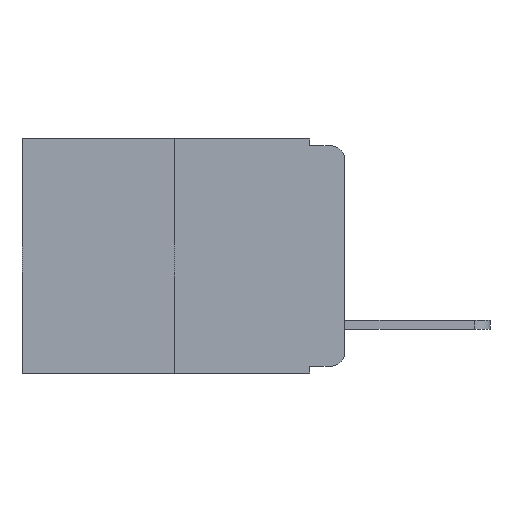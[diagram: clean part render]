
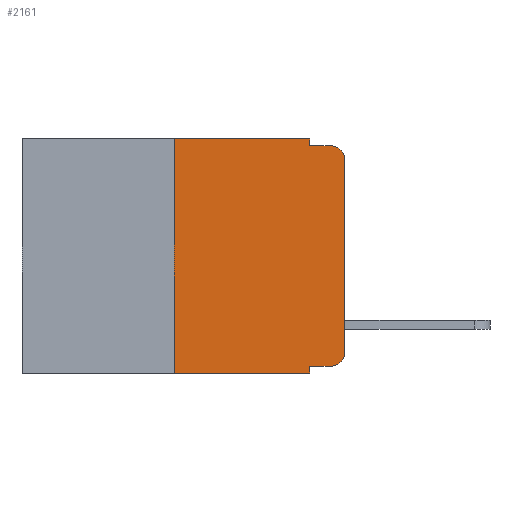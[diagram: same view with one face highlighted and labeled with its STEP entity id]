
A CAD part, left-side view. The second image highlights one B-rep face of the part: STEP entity #2161.
In plain terms, the highlighted planar face has unit normal (-1, 0, 0).
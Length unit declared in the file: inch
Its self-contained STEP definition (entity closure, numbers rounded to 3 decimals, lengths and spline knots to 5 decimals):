
#366 = VERTEX_POINT ( 'NONE', #12138 ) ;
#559 = DIRECTION ( 'NONE',  ( 0., -1., 0. ) ) ;
#1213 = VECTOR ( 'NONE', #559, 39.37008 ) ;
#1347 = CARTESIAN_POINT ( 'NONE',  ( 0., 0.051, -0.01 ) ) ;
#1395 = CARTESIAN_POINT ( 'NONE',  ( 0., 0.02, -0.03 ) ) ;
#1619 = CARTESIAN_POINT ( 'NONE',  ( 0., 0.25, 0. ) ) ;
#1720 = LINE ( 'NONE', #11743, #8694 ) ;
#1754 = DIRECTION ( 'NONE',  ( 1., 0., 0. ) ) ;
#1811 = LINE ( 'NONE', #12158, #14502 ) ;
#1887 = CARTESIAN_POINT ( 'NONE',  ( 0., 0.02, -0.01 ) ) ;
#2161 = ADVANCED_FACE ( 'NONE', ( #7133 ), #8651, .F. ) ;
#2276 = DIRECTION ( 'NONE',  ( -1., 0., 0. ) ) ;
#2451 = VECTOR ( 'NONE', #3055, 39.37008 ) ;
#2635 = DIRECTION ( 'NONE',  ( 0., 0., -1. ) ) ;
#2813 = DIRECTION ( 'NONE',  ( 0., 0., -1. ) ) ;
#2818 = VECTOR ( 'NONE', #8005, 39.37008 ) ;
#3055 = DIRECTION ( 'NONE',  ( 0., 0., -1. ) ) ;
#3097 = EDGE_CURVE ( 'NONE', #13874, #5766, #4501, .T. ) ;
#3122 = ORIENTED_EDGE ( 'NONE', *, *, #5126, .T. ) ;
#3855 = VECTOR ( 'NONE', #10540, 39.37008 ) ;
#3976 = EDGE_CURVE ( 'NONE', #11654, #7287, #7763, .T. ) ;
#4277 = VECTOR ( 'NONE', #8811, 39.37008 ) ;
#4360 = DIRECTION ( 'NONE',  ( 0., 0., 1. ) ) ;
#4501 = LINE ( 'NONE', #1347, #1213 ) ;
#4896 = VERTEX_POINT ( 'NONE', #12552 ) ;
#5019 = AXIS2_PLACEMENT_3D ( 'NONE', #7340, #1754, #2813 ) ;
#5088 = CARTESIAN_POINT ( 'NONE',  ( 0., 0.473, -0.343 ) ) ;
#5126 = EDGE_CURVE ( 'NONE', #366, #11071, #10782, .T. ) ;
#5196 = CARTESIAN_POINT ( 'NONE',  ( 0., 0.25, -0.343 ) ) ;
#5318 = EDGE_CURVE ( 'NONE', #11071, #7350, #14222, .T. ) ;
#5589 = AXIS2_PLACEMENT_3D ( 'NONE', #1395, #10014, #2635 ) ;
#5659 = ORIENTED_EDGE ( 'NONE', *, *, #10880, .F. ) ;
#5766 = VERTEX_POINT ( 'NONE', #1887 ) ;
#6203 = ORIENTED_EDGE ( 'NONE', *, *, #13486, .T. ) ;
#6761 = CARTESIAN_POINT ( 'NONE',  ( 0., 0.051, 0. ) ) ;
#7133 = FACE_OUTER_BOUND ( 'NONE', #9775, .T. ) ;
#7287 = VERTEX_POINT ( 'NONE', #13765 ) ;
#7340 = CARTESIAN_POINT ( 'NONE',  ( 0., 0.473, 0. ) ) ;
#7350 = VERTEX_POINT ( 'NONE', #8985 ) ;
#7395 = ORIENTED_EDGE ( 'NONE', *, *, #3976, .F. ) ;
#7576 = LINE ( 'NONE', #5088, #4277 ) ;
#7763 = LINE ( 'NONE', #8112, #13898 ) ;
#7936 = CIRCLE ( 'NONE', #5589, 0.02 ) ;
#8005 = DIRECTION ( 'NONE',  ( 0., 0., -1. ) ) ;
#8017 = EDGE_CURVE ( 'NONE', #366, #9516, #12270, .T. ) ;
#8112 = CARTESIAN_POINT ( 'NONE',  ( 0., 0.473, 0. ) ) ;
#8351 = ORIENTED_EDGE ( 'NONE', *, *, #12646, .T. ) ;
#8651 = PLANE ( 'NONE',  #5019 ) ;
#8694 = VECTOR ( 'NONE', #4360, 39.37008 ) ;
#8746 = AXIS2_PLACEMENT_3D ( 'NONE', #9675, #2276, #10911 ) ;
#8811 = DIRECTION ( 'NONE',  ( 0., -1., 0. ) ) ;
#8833 = ORIENTED_EDGE ( 'NONE', *, *, #8017, .F. ) ;
#8985 = CARTESIAN_POINT ( 'NONE',  ( 0., 0., -0.313 ) ) ;
#9018 = LINE ( 'NONE', #6761, #2451 ) ;
#9309 = CARTESIAN_POINT ( 'NONE',  ( 0., 0.051, -0.333 ) ) ;
#9392 = CARTESIAN_POINT ( 'NONE',  ( 0., 0.051, -0.343 ) ) ;
#9422 = EDGE_CURVE ( 'NONE', #7287, #13874, #9018, .T. ) ;
#9516 = VERTEX_POINT ( 'NONE', #9392 ) ;
#9675 = CARTESIAN_POINT ( 'NONE',  ( 0., 0.02, -0.313 ) ) ;
#9775 = EDGE_LOOP ( 'NONE', ( #6203, #12800, #14505, #10079, #7395, #5659, #8351, #8833, #3122, #11306 ) ) ;
#10014 = DIRECTION ( 'NONE',  ( -1., 0., 0. ) ) ;
#10079 = ORIENTED_EDGE ( 'NONE', *, *, #9422, .F. ) ;
#10540 = DIRECTION ( 'NONE',  ( 0., -1., 0. ) ) ;
#10782 = LINE ( 'NONE', #9309, #3855 ) ;
#10880 = EDGE_CURVE ( 'NONE', #11084, #11654, #1811, .T. ) ;
#10911 = DIRECTION ( 'NONE',  ( 0., 0., -1. ) ) ;
#11071 = VERTEX_POINT ( 'NONE', #11347 ) ;
#11084 = VERTEX_POINT ( 'NONE', #5196 ) ;
#11306 = ORIENTED_EDGE ( 'NONE', *, *, #5318, .T. ) ;
#11347 = CARTESIAN_POINT ( 'NONE',  ( 0., 0.02, -0.333 ) ) ;
#11654 = VERTEX_POINT ( 'NONE', #1619 ) ;
#11743 = CARTESIAN_POINT ( 'NONE',  ( 0., 0., 0. ) ) ;
#12138 = CARTESIAN_POINT ( 'NONE',  ( 0., 0.051, -0.333 ) ) ;
#12158 = CARTESIAN_POINT ( 'NONE',  ( 0., 0.25, 0. ) ) ;
#12270 = LINE ( 'NONE', #15317, #2818 ) ;
#12552 = CARTESIAN_POINT ( 'NONE',  ( 0., 0., -0.03 ) ) ;
#12593 = CARTESIAN_POINT ( 'NONE',  ( 0., 0.051, -0.01 ) ) ;
#12646 = EDGE_CURVE ( 'NONE', #11084, #9516, #7576, .T. ) ;
#12800 = ORIENTED_EDGE ( 'NONE', *, *, #15795, .T. ) ;
#13055 = DIRECTION ( 'NONE',  ( 0., -1., 0. ) ) ;
#13486 = EDGE_CURVE ( 'NONE', #7350, #4896, #1720, .T. ) ;
#13765 = CARTESIAN_POINT ( 'NONE',  ( 0., 0.051, 0. ) ) ;
#13874 = VERTEX_POINT ( 'NONE', #12593 ) ;
#13898 = VECTOR ( 'NONE', #13055, 39.37008 ) ;
#14222 = CIRCLE ( 'NONE', #8746, 0.02 ) ;
#14502 = VECTOR ( 'NONE', #15791, 39.37008 ) ;
#14505 = ORIENTED_EDGE ( 'NONE', *, *, #3097, .F. ) ;
#15317 = CARTESIAN_POINT ( 'NONE',  ( 0., 0.051, 0. ) ) ;
#15791 = DIRECTION ( 'NONE',  ( 0., 0., 1. ) ) ;
#15795 = EDGE_CURVE ( 'NONE', #4896, #5766, #7936, .T. ) ;
